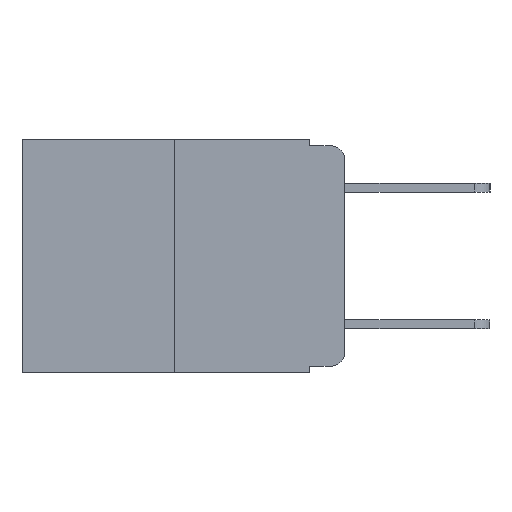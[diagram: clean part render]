
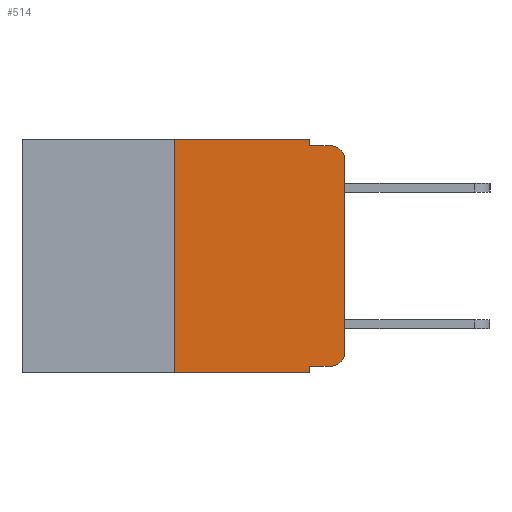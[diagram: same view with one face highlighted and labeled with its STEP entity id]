
A CAD part, left-side view. The second image highlights one B-rep face of the part: STEP entity #514.
In plain terms, the highlighted planar face has unit normal (-1, 0, 0).
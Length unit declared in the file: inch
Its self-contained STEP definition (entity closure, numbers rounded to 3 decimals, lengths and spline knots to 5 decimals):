
#76 = ORIENTED_EDGE ( 'NONE', *, *, #5631, .F. ) ;
#77 = ORIENTED_EDGE ( 'NONE', *, *, #7506, .T. ) ;
#152 = CARTESIAN_POINT ( 'NONE',  ( 0., 0.051, 0. ) ) ;
#383 = VERTEX_POINT ( 'NONE', #2855 ) ;
#440 = CARTESIAN_POINT ( 'NONE',  ( 0., 0.473, 0. ) ) ;
#514 = ADVANCED_FACE ( 'NONE', ( #944 ), #2184, .F. ) ;
#563 = VERTEX_POINT ( 'NONE', #6867 ) ;
#653 = DIRECTION ( 'NONE',  ( 0., 0., -1. ) ) ;
#720 = CARTESIAN_POINT ( 'NONE',  ( 0., 0.051, -0.333 ) ) ;
#850 = DIRECTION ( 'NONE',  ( 0., 0., 1. ) ) ;
#923 = VERTEX_POINT ( 'NONE', #9796 ) ;
#944 = FACE_OUTER_BOUND ( 'NONE', #4267, .T. ) ;
#1066 = ORIENTED_EDGE ( 'NONE', *, *, #3140, .F. ) ;
#1162 = CARTESIAN_POINT ( 'NONE',  ( 0., 0., 0. ) ) ;
#1168 = ORIENTED_EDGE ( 'NONE', *, *, #11269, .T. ) ;
#1405 = CARTESIAN_POINT ( 'NONE',  ( 0., 0.051, -0.01 ) ) ;
#1644 = DIRECTION ( 'NONE',  ( 0., -1., 0. ) ) ;
#1725 = EDGE_CURVE ( 'NONE', #12004, #7146, #4140, .T. ) ;
#1929 = VECTOR ( 'NONE', #1644, 39.37008 ) ;
#2017 = LINE ( 'NONE', #4005, #11341 ) ;
#2135 = AXIS2_PLACEMENT_3D ( 'NONE', #4422, #10533, #5408 ) ;
#2140 = CARTESIAN_POINT ( 'NONE',  ( 0., 0.473, 0. ) ) ;
#2150 = DIRECTION ( 'NONE',  ( 0., 0., -1. ) ) ;
#2184 = PLANE ( 'NONE',  #2236 ) ;
#2236 = AXIS2_PLACEMENT_3D ( 'NONE', #2140, #6984, #2150 ) ;
#2244 = DIRECTION ( 'NONE',  ( 0., 0., -1. ) ) ;
#2490 = EDGE_CURVE ( 'NONE', #6167, #12004, #10419, .T. ) ;
#2769 = DIRECTION ( 'NONE',  ( 0., -1., 0. ) ) ;
#2855 = CARTESIAN_POINT ( 'NONE',  ( 0., 0.25, -0.343 ) ) ;
#2912 = CARTESIAN_POINT ( 'NONE',  ( 0., 0., -0.313 ) ) ;
#3140 = EDGE_CURVE ( 'NONE', #6167, #923, #7385, .T. ) ;
#3320 = VECTOR ( 'NONE', #11795, 39.37008 ) ;
#3532 = VECTOR ( 'NONE', #6205, 39.37008 ) ;
#3554 = VECTOR ( 'NONE', #2769, 39.37008 ) ;
#3824 = EDGE_CURVE ( 'NONE', #383, #563, #2017, .T. ) ;
#4005 = CARTESIAN_POINT ( 'NONE',  ( 0., 0.25, 0. ) ) ;
#4008 = CARTESIAN_POINT ( 'NONE',  ( 0., 0.02, -0.333 ) ) ;
#4035 = ORIENTED_EDGE ( 'NONE', *, *, #6925, .T. ) ;
#4140 = CIRCLE ( 'NONE', #7459, 0.02 ) ;
#4175 = ORIENTED_EDGE ( 'NONE', *, *, #5749, .F. ) ;
#4267 = EDGE_LOOP ( 'NONE', ( #77, #4035, #4563, #4175, #76, #9320, #1168, #1066, #6050, #5106 ) ) ;
#4303 = LINE ( 'NONE', #7421, #1929 ) ;
#4409 = VERTEX_POINT ( 'NONE', #10873 ) ;
#4422 = CARTESIAN_POINT ( 'NONE',  ( 0., 0.02, -0.03 ) ) ;
#4563 = ORIENTED_EDGE ( 'NONE', *, *, #6355, .F. ) ;
#5030 = VECTOR ( 'NONE', #8703, 39.37008 ) ;
#5106 = ORIENTED_EDGE ( 'NONE', *, *, #1725, .T. ) ;
#5408 = DIRECTION ( 'NONE',  ( 0., 0., -1. ) ) ;
#5499 = VERTEX_POINT ( 'NONE', #152 ) ;
#5631 = EDGE_CURVE ( 'NONE', #563, #5499, #9956, .T. ) ;
#5703 = CARTESIAN_POINT ( 'NONE',  ( 0., 0.02, -0.313 ) ) ;
#5749 = EDGE_CURVE ( 'NONE', #5499, #10413, #6641, .T. ) ;
#5924 = LINE ( 'NONE', #1162, #3532 ) ;
#5935 = VERTEX_POINT ( 'NONE', #11125 ) ;
#6050 = ORIENTED_EDGE ( 'NONE', *, *, #2490, .T. ) ;
#6167 = VERTEX_POINT ( 'NONE', #8042 ) ;
#6205 = DIRECTION ( 'NONE',  ( 0., 0., 1. ) ) ;
#6355 = EDGE_CURVE ( 'NONE', #10413, #4409, #4303, .T. ) ;
#6524 = DIRECTION ( 'NONE',  ( 0., -1., 0. ) ) ;
#6641 = LINE ( 'NONE', #11768, #10896 ) ;
#6867 = CARTESIAN_POINT ( 'NONE',  ( 0., 0.25, 0. ) ) ;
#6925 = EDGE_CURVE ( 'NONE', #5935, #4409, #11010, .T. ) ;
#6984 = DIRECTION ( 'NONE',  ( 1., 0., 0. ) ) ;
#7146 = VERTEX_POINT ( 'NONE', #2912 ) ;
#7385 = LINE ( 'NONE', #10320, #5030 ) ;
#7421 = CARTESIAN_POINT ( 'NONE',  ( 0., 0.051, -0.01 ) ) ;
#7459 = AXIS2_PLACEMENT_3D ( 'NONE', #5703, #7842, #2244 ) ;
#7506 = EDGE_CURVE ( 'NONE', #7146, #5935, #5924, .T. ) ;
#7842 = DIRECTION ( 'NONE',  ( -1., 0., 0. ) ) ;
#7987 = VECTOR ( 'NONE', #6524, 39.37008 ) ;
#8042 = CARTESIAN_POINT ( 'NONE',  ( 0., 0.051, -0.333 ) ) ;
#8703 = DIRECTION ( 'NONE',  ( 0., 0., -1. ) ) ;
#9320 = ORIENTED_EDGE ( 'NONE', *, *, #3824, .F. ) ;
#9796 = CARTESIAN_POINT ( 'NONE',  ( 0., 0.051, -0.343 ) ) ;
#9956 = LINE ( 'NONE', #440, #7987 ) ;
#10320 = CARTESIAN_POINT ( 'NONE',  ( 0., 0.051, 0. ) ) ;
#10413 = VERTEX_POINT ( 'NONE', #1405 ) ;
#10419 = LINE ( 'NONE', #720, #3320 ) ;
#10533 = DIRECTION ( 'NONE',  ( -1., 0., 0. ) ) ;
#10618 = LINE ( 'NONE', #11641, #3554 ) ;
#10873 = CARTESIAN_POINT ( 'NONE',  ( 0., 0.02, -0.01 ) ) ;
#10896 = VECTOR ( 'NONE', #653, 39.37008 ) ;
#11010 = CIRCLE ( 'NONE', #2135, 0.02 ) ;
#11125 = CARTESIAN_POINT ( 'NONE',  ( 0., 0., -0.03 ) ) ;
#11269 = EDGE_CURVE ( 'NONE', #383, #923, #10618, .T. ) ;
#11341 = VECTOR ( 'NONE', #850, 39.37008 ) ;
#11641 = CARTESIAN_POINT ( 'NONE',  ( 0., 0.473, -0.343 ) ) ;
#11768 = CARTESIAN_POINT ( 'NONE',  ( 0., 0.051, 0. ) ) ;
#11795 = DIRECTION ( 'NONE',  ( 0., -1., 0. ) ) ;
#12004 = VERTEX_POINT ( 'NONE', #4008 ) ;
